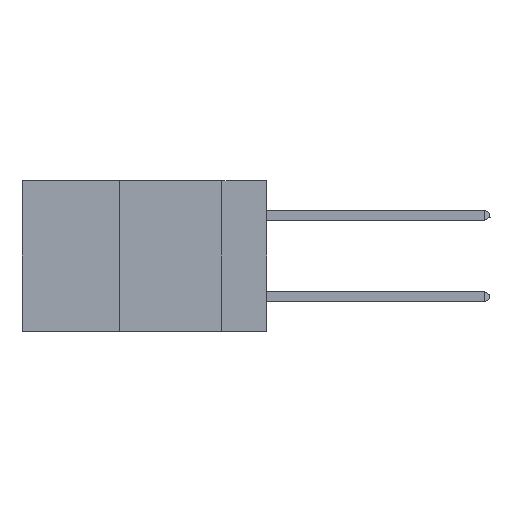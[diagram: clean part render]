
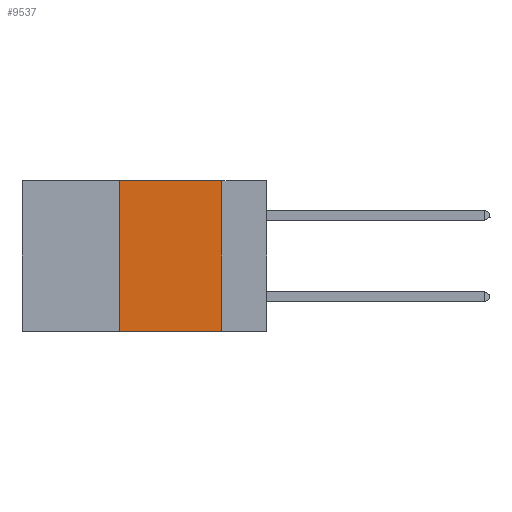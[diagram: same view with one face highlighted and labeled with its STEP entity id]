
A CAD part, left-side view. The second image highlights one B-rep face of the part: STEP entity #9537.
In plain terms, the highlighted planar face has unit normal (-1, 0, 0).
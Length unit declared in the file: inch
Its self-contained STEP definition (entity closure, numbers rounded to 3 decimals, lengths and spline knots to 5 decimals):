
#110 = CARTESIAN_POINT ( 'NONE',  ( 0., 0.11, 0. ) ) ;
#130 = EDGE_CURVE ( 'NONE', #10952, #8419, #10062, .T. ) ;
#238 = EDGE_CURVE ( 'NONE', #7371, #1855, #4623, .T. ) ;
#1411 = VECTOR ( 'NONE', #10400, 39.37008 ) ;
#1534 = VECTOR ( 'NONE', #4157, 39.37008 ) ;
#1855 = VERTEX_POINT ( 'NONE', #5362 ) ;
#2029 = DIRECTION ( 'NONE',  ( 0., 0., 1. ) ) ;
#2999 = ORIENTED_EDGE ( 'NONE', *, *, #130, .F. ) ;
#3534 = CARTESIAN_POINT ( 'NONE',  ( 0., 0.6, 0. ) ) ;
#3605 = CARTESIAN_POINT ( 'NONE',  ( 0., 0.36, -0.37 ) ) ;
#3761 = CARTESIAN_POINT ( 'NONE',  ( 0., 0.36, 0. ) ) ;
#4157 = DIRECTION ( 'NONE',  ( 0., -1., 0. ) ) ;
#4507 = CARTESIAN_POINT ( 'NONE',  ( 0., 0.11, 0. ) ) ;
#4623 = LINE ( 'NONE', #3761, #7028 ) ;
#5362 = CARTESIAN_POINT ( 'NONE',  ( 0., 0.36, 0. ) ) ;
#5538 = ORIENTED_EDGE ( 'NONE', *, *, #238, .F. ) ;
#5931 = EDGE_CURVE ( 'NONE', #1855, #10952, #10407, .T. ) ;
#6045 = CARTESIAN_POINT ( 'NONE',  ( 0., 0.6, 0. ) ) ;
#6159 = DIRECTION ( 'NONE',  ( 1., 0., 0. ) ) ;
#6221 = DIRECTION ( 'NONE',  ( 0., 0., -1. ) ) ;
#6752 = CARTESIAN_POINT ( 'NONE',  ( 0., 0.6, -0.37 ) ) ;
#6921 = FACE_OUTER_BOUND ( 'NONE', #10585, .T. ) ;
#7028 = VECTOR ( 'NONE', #2029, 39.37008 ) ;
#7371 = VERTEX_POINT ( 'NONE', #3605 ) ;
#8419 = VERTEX_POINT ( 'NONE', #10965 ) ;
#8942 = ORIENTED_EDGE ( 'NONE', *, *, #9421, .T. ) ;
#9296 = ORIENTED_EDGE ( 'NONE', *, *, #5931, .F. ) ;
#9421 = EDGE_CURVE ( 'NONE', #7371, #8419, #10286, .T. ) ;
#9537 = ADVANCED_FACE ( 'NONE', ( #6921 ), #10460, .F. ) ;
#10062 = LINE ( 'NONE', #110, #10728 ) ;
#10286 = LINE ( 'NONE', #6752, #1411 ) ;
#10400 = DIRECTION ( 'NONE',  ( 0., -1., 0. ) ) ;
#10407 = LINE ( 'NONE', #3534, #1534 ) ;
#10460 = PLANE ( 'NONE',  #11211 ) ;
#10585 = EDGE_LOOP ( 'NONE', ( #2999, #9296, #5538, #8942 ) ) ;
#10728 = VECTOR ( 'NONE', #10822, 39.37008 ) ;
#10822 = DIRECTION ( 'NONE',  ( 0., 0., -1. ) ) ;
#10952 = VERTEX_POINT ( 'NONE', #4507 ) ;
#10965 = CARTESIAN_POINT ( 'NONE',  ( 0., 0.11, -0.37 ) ) ;
#11211 = AXIS2_PLACEMENT_3D ( 'NONE', #6045, #6159, #6221 ) ;
